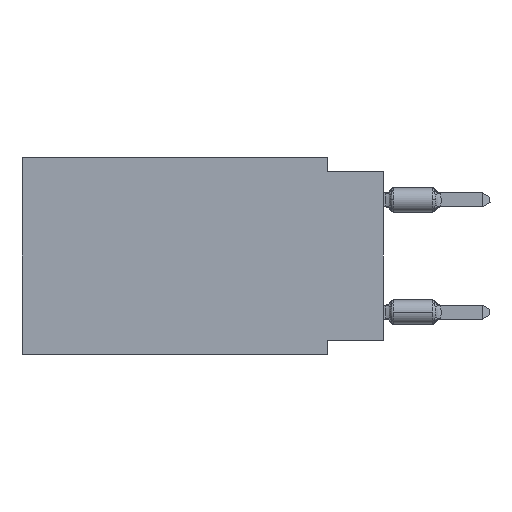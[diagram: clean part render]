
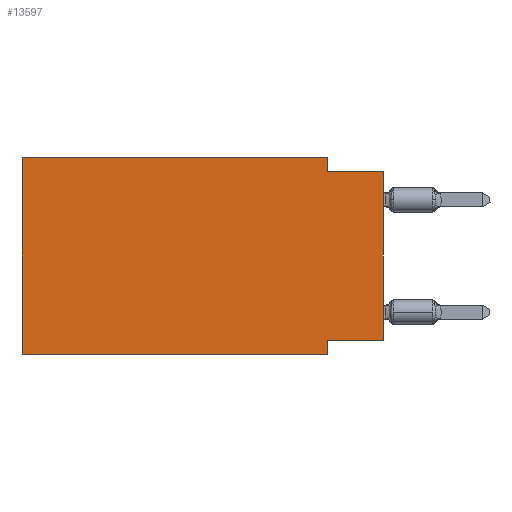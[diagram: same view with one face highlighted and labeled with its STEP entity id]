
A CAD part, left-side view. The second image highlights one B-rep face of the part: STEP entity #13597.
In plain terms, the highlighted planar face has unit normal (-1, 0, 0).
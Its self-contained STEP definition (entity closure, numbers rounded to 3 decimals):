
#582 = AXIS2_PLACEMENT_3D ( 'NONE', #13993, #18231, #22113 ) ;
#631 = CARTESIAN_POINT ( 'NONE',  ( 0., 16.383, 0. ) ) ;
#771 = CARTESIAN_POINT ( 'NONE',  ( 0., 2.54, 0. ) ) ;
#1164 = CARTESIAN_POINT ( 'NONE',  ( 0., 0., 0. ) ) ;
#1288 = VERTEX_POINT ( 'NONE', #24516 ) ;
#1510 = ORIENTED_EDGE ( 'NONE', *, *, #15874, .F. ) ;
#1712 = VERTEX_POINT ( 'NONE', #4416 ) ;
#2343 = DIRECTION ( 'NONE',  ( 0., 0., -1. ) ) ;
#2498 = CARTESIAN_POINT ( 'NONE',  ( 0., 2.54, -0.635 ) ) ;
#3404 = LINE ( 'NONE', #21886, #15251 ) ;
#3459 = DIRECTION ( 'NONE',  ( 0., -1., 0. ) ) ;
#3814 = VERTEX_POINT ( 'NONE', #5252 ) ;
#3974 = EDGE_CURVE ( 'NONE', #3814, #23405, #20145, .T. ) ;
#4416 = CARTESIAN_POINT ( 'NONE',  ( 0., 2.54, -8.89 ) ) ;
#4840 = VERTEX_POINT ( 'NONE', #17612 ) ;
#4961 = EDGE_CURVE ( 'NONE', #10938, #1288, #3404, .T. ) ;
#5252 = CARTESIAN_POINT ( 'NONE',  ( 0., 0., -8.255 ) ) ;
#5524 = CARTESIAN_POINT ( 'NONE',  ( 0., 0., -8.255 ) ) ;
#6253 = VECTOR ( 'NONE', #10500, 1000. ) ;
#6487 = CARTESIAN_POINT ( 'NONE',  ( 0., 2.54, -8.89 ) ) ;
#6629 = DIRECTION ( 'NONE',  ( 0., 0., -1. ) ) ;
#7388 = DIRECTION ( 'NONE',  ( 0., 1., 0. ) ) ;
#7514 = EDGE_CURVE ( 'NONE', #12237, #10938, #19106, .T. ) ;
#7742 = CARTESIAN_POINT ( 'NONE',  ( 0., 2.54, 0. ) ) ;
#7878 = ORIENTED_EDGE ( 'NONE', *, *, #14176, .T. ) ;
#7918 = VECTOR ( 'NONE', #6629, 1000. ) ;
#9057 = VECTOR ( 'NONE', #3459, 1000. ) ;
#9271 = LINE ( 'NONE', #1164, #23069 ) ;
#9578 = ORIENTED_EDGE ( 'NONE', *, *, #4961, .F. ) ;
#10453 = ORIENTED_EDGE ( 'NONE', *, *, #19652, .F. ) ;
#10500 = DIRECTION ( 'NONE',  ( 0., -1., 0. ) ) ;
#10938 = VERTEX_POINT ( 'NONE', #2498 ) ;
#12237 = VERTEX_POINT ( 'NONE', #7742 ) ;
#12402 = PLANE ( 'NONE',  #582 ) ;
#13597 = ADVANCED_FACE ( 'NONE', ( #14251 ), #12402, .F. ) ;
#13891 = EDGE_CURVE ( 'NONE', #23396, #1712, #23660, .T. ) ;
#13993 = CARTESIAN_POINT ( 'NONE',  ( 0., 16.383, 0. ) ) ;
#14176 = EDGE_CURVE ( 'NONE', #3814, #1288, #9271, .T. ) ;
#14251 = FACE_OUTER_BOUND ( 'NONE', #21442, .T. ) ;
#15251 = VECTOR ( 'NONE', #24788, 1000. ) ;
#15336 = EDGE_CURVE ( 'NONE', #4840, #12237, #18464, .T. ) ;
#15874 = EDGE_CURVE ( 'NONE', #23405, #1712, #20576, .T. ) ;
#15951 = CARTESIAN_POINT ( 'NONE',  ( 0., 16.383, 0. ) ) ;
#16937 = CARTESIAN_POINT ( 'NONE',  ( 0., 2.54, -8.255 ) ) ;
#17076 = VECTOR ( 'NONE', #7388, 1000. ) ;
#17612 = CARTESIAN_POINT ( 'NONE',  ( 0., 16.383, 0. ) ) ;
#17789 = VECTOR ( 'NONE', #20582, 1000. ) ;
#18231 = DIRECTION ( 'NONE',  ( 1., 0., 0. ) ) ;
#18464 = LINE ( 'NONE', #15951, #6253 ) ;
#19106 = LINE ( 'NONE', #771, #7918 ) ;
#19248 = ORIENTED_EDGE ( 'NONE', *, *, #7514, .F. ) ;
#19652 = EDGE_CURVE ( 'NONE', #23396, #4840, #20455, .T. ) ;
#20145 = LINE ( 'NONE', #5524, #17076 ) ;
#20455 = LINE ( 'NONE', #631, #17789 ) ;
#20576 = LINE ( 'NONE', #6487, #21141 ) ;
#20582 = DIRECTION ( 'NONE',  ( 0., 0., 1. ) ) ;
#21141 = VECTOR ( 'NONE', #2343, 1000. ) ;
#21442 = EDGE_LOOP ( 'NONE', ( #7878, #9578, #19248, #22176, #10453, #25313, #1510, #26070 ) ) ;
#21687 = CARTESIAN_POINT ( 'NONE',  ( 0., 16.383, -8.89 ) ) ;
#21886 = CARTESIAN_POINT ( 'NONE',  ( 0., 0., -0.635 ) ) ;
#22113 = DIRECTION ( 'NONE',  ( 0., 0., -1. ) ) ;
#22176 = ORIENTED_EDGE ( 'NONE', *, *, #15336, .F. ) ;
#23069 = VECTOR ( 'NONE', #23627, 1000. ) ;
#23396 = VERTEX_POINT ( 'NONE', #25177 ) ;
#23405 = VERTEX_POINT ( 'NONE', #16937 ) ;
#23627 = DIRECTION ( 'NONE',  ( 0., 0., 1. ) ) ;
#23660 = LINE ( 'NONE', #21687, #9057 ) ;
#24516 = CARTESIAN_POINT ( 'NONE',  ( 0., 0., -0.635 ) ) ;
#24788 = DIRECTION ( 'NONE',  ( 0., -1., 0. ) ) ;
#25177 = CARTESIAN_POINT ( 'NONE',  ( 0., 16.383, -8.89 ) ) ;
#25313 = ORIENTED_EDGE ( 'NONE', *, *, #13891, .T. ) ;
#26070 = ORIENTED_EDGE ( 'NONE', *, *, #3974, .F. ) ;
